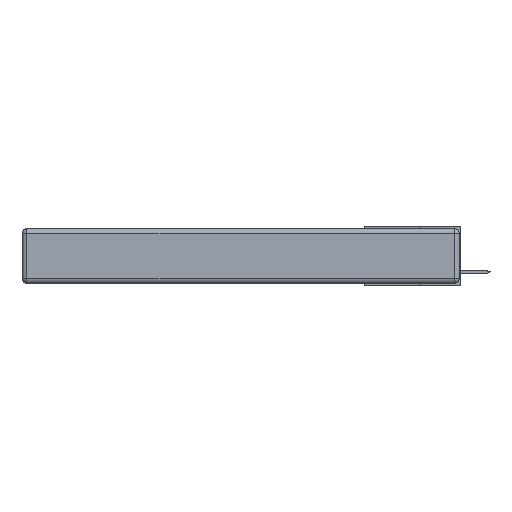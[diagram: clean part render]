
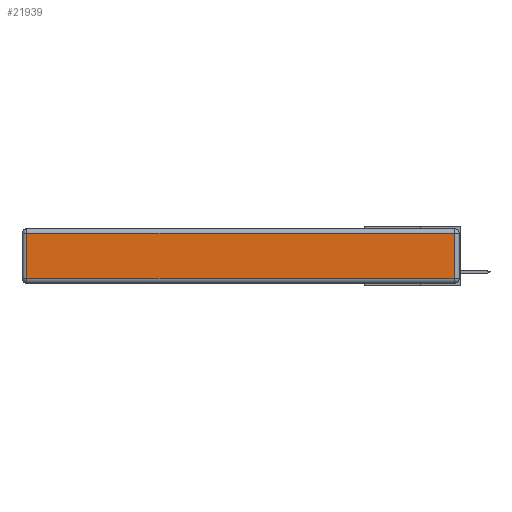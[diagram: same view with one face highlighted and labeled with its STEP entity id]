
A CAD part, left-side view. The second image highlights one B-rep face of the part: STEP entity #21939.
In plain terms, the highlighted planar face has unit normal (-1, 0, 0).
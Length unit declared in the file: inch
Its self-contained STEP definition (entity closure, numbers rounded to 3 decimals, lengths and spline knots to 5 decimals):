
#318 = VERTEX_POINT ( 'NONE', #4913 ) ;
#1431 = DIRECTION ( 'NONE',  ( 0., -1., 0. ) ) ;
#1750 = VECTOR ( 'NONE', #2998, 39.37008 ) ;
#2998 = DIRECTION ( 'NONE',  ( 0., 1., 0. ) ) ;
#3232 = CARTESIAN_POINT ( 'NONE',  ( 0., 2.72, -0.313 ) ) ;
#4359 = AXIS2_PLACEMENT_3D ( 'NONE', #5700, #21449, #28263 ) ;
#4913 = CARTESIAN_POINT ( 'NONE',  ( 0., 0.03, -0.313 ) ) ;
#5700 = CARTESIAN_POINT ( 'NONE',  ( 0., 0., -0.343 ) ) ;
#7043 = EDGE_CURVE ( 'NONE', #18893, #25394, #17602, .T. ) ;
#8248 = LINE ( 'NONE', #13361, #24842 ) ;
#9408 = DIRECTION ( 'NONE',  ( 0., 0., 1. ) ) ;
#9987 = EDGE_CURVE ( 'NONE', #25394, #23974, #8248, .T. ) ;
#10705 = DIRECTION ( 'NONE',  ( 0., 0., -1. ) ) ;
#11620 = FACE_OUTER_BOUND ( 'NONE', #20528, .T. ) ;
#11673 = ORIENTED_EDGE ( 'NONE', *, *, #7043, .T. ) ;
#13361 = CARTESIAN_POINT ( 'NONE',  ( 0., 2.72, -0.343 ) ) ;
#13681 = EDGE_CURVE ( 'NONE', #318, #18893, #22397, .T. ) ;
#17081 = VECTOR ( 'NONE', #9408, 39.37008 ) ;
#17602 = LINE ( 'NONE', #27578, #1750 ) ;
#17760 = ORIENTED_EDGE ( 'NONE', *, *, #9987, .T. ) ;
#18354 = ORIENTED_EDGE ( 'NONE', *, *, #13681, .T. ) ;
#18654 = CARTESIAN_POINT ( 'NONE',  ( 0., 0.03, -0.343 ) ) ;
#18738 = CARTESIAN_POINT ( 'NONE',  ( 0., 0.03, -0.03 ) ) ;
#18893 = VERTEX_POINT ( 'NONE', #18738 ) ;
#19166 = PLANE ( 'NONE',  #4359 ) ;
#20528 = EDGE_LOOP ( 'NONE', ( #23721, #18354, #11673, #17760 ) ) ;
#21449 = DIRECTION ( 'NONE',  ( -1., 0., 0. ) ) ;
#21939 = ADVANCED_FACE ( 'NONE', ( #11620 ), #19166, .T. ) ;
#22397 = LINE ( 'NONE', #18654, #17081 ) ;
#23515 = CARTESIAN_POINT ( 'NONE',  ( 0., 0., -0.313 ) ) ;
#23721 = ORIENTED_EDGE ( 'NONE', *, *, #24237, .T. ) ;
#23974 = VERTEX_POINT ( 'NONE', #3232 ) ;
#24237 = EDGE_CURVE ( 'NONE', #23974, #318, #25702, .T. ) ;
#24842 = VECTOR ( 'NONE', #10705, 39.37008 ) ;
#25394 = VERTEX_POINT ( 'NONE', #25634 ) ;
#25634 = CARTESIAN_POINT ( 'NONE',  ( 0., 2.72, -0.03 ) ) ;
#25702 = LINE ( 'NONE', #23515, #28532 ) ;
#27578 = CARTESIAN_POINT ( 'NONE',  ( 0., 2.75, -0.03 ) ) ;
#28263 = DIRECTION ( 'NONE',  ( 0., 0., 1. ) ) ;
#28532 = VECTOR ( 'NONE', #1431, 39.37008 ) ;
